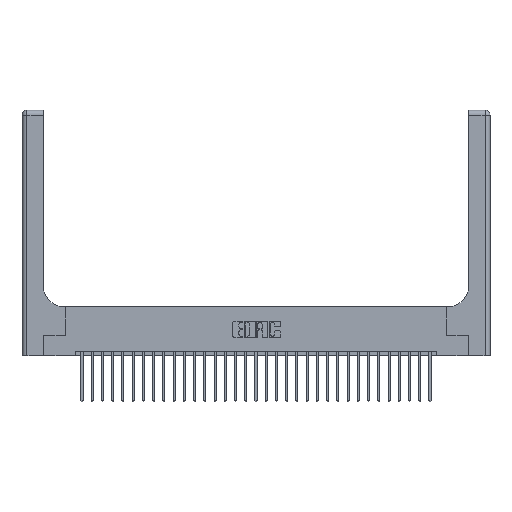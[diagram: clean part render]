
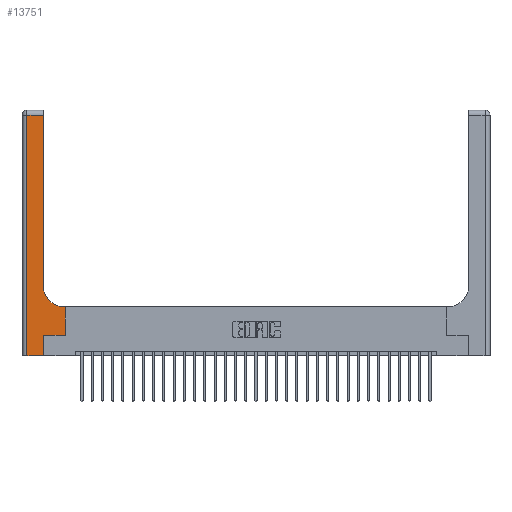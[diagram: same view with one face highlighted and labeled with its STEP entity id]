
A CAD part, top view. The second image highlights one B-rep face of the part: STEP entity #13751.
In plain terms, the highlighted planar face has unit normal (0, 0, 1).
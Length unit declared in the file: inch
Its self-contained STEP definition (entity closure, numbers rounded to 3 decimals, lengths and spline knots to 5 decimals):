
#212 = ORIENTED_EDGE ( 'NONE', *, *, #24034, .T. ) ;
#1287 = EDGE_CURVE ( 'NONE', #4562, #25562, #9006, .T. ) ;
#1289 = VERTEX_POINT ( 'NONE', #25247 ) ;
#1395 = LINE ( 'NONE', #23115, #12663 ) ;
#1479 = ORIENTED_EDGE ( 'NONE', *, *, #27696, .T. ) ;
#1590 = ORIENTED_EDGE ( 'NONE', *, *, #26799, .T. ) ;
#1836 = EDGE_CURVE ( 'NONE', #21965, #18299, #26508, .T. ) ;
#2202 = CARTESIAN_POINT ( 'NONE',  ( 0.265, 0.25, 0.37 ) ) ;
#2349 = CARTESIAN_POINT ( 'NONE',  ( 0.06, 3., 0.37 ) ) ;
#2582 = ORIENTED_EDGE ( 'NONE', *, *, #17520, .T. ) ;
#3623 = ORIENTED_EDGE ( 'NONE', *, *, #25007, .T. ) ;
#3646 = CARTESIAN_POINT ( 'NONE',  ( 0.26, 3., 0.37 ) ) ;
#4562 = VERTEX_POINT ( 'NONE', #13557 ) ;
#5045 = LINE ( 'NONE', #2202, #22227 ) ;
#6252 = VERTEX_POINT ( 'NONE', #26612 ) ;
#6631 = EDGE_CURVE ( 'NONE', #1289, #6252, #18852, .T. ) ;
#6701 = DIRECTION ( 'NONE',  ( -1., 0., 0. ) ) ;
#6970 = VERTEX_POINT ( 'NONE', #17589 ) ;
#7402 = VECTOR ( 'NONE', #24679, 39.37008 ) ;
#7722 = DIRECTION ( 'NONE',  ( -1., 0., 0. ) ) ;
#8381 = DIRECTION ( 'NONE',  ( 0., 1., 0. ) ) ;
#8874 = VECTOR ( 'NONE', #19565, 39.37008 ) ;
#9006 = LINE ( 'NONE', #11857, #16437 ) ;
#9438 = CARTESIAN_POINT ( 'NONE',  ( 0.06, 2.94, 0.37 ) ) ;
#9473 = CARTESIAN_POINT ( 'NONE',  ( 0.51, 0.6, 0.37 ) ) ;
#10012 = FACE_OUTER_BOUND ( 'NONE', #28015, .T. ) ;
#10617 = CARTESIAN_POINT ( 'NONE',  ( 0.528, 0.25, 0.37 ) ) ;
#10972 = CARTESIAN_POINT ( 'NONE',  ( 0., 2.94, 0.37 ) ) ;
#11434 = VECTOR ( 'NONE', #20041, 39.37008 ) ;
#11857 = CARTESIAN_POINT ( 'NONE',  ( 0.26, 0.6, 0.37 ) ) ;
#11878 = CIRCLE ( 'NONE', #12077, 0.25 ) ;
#11880 = CARTESIAN_POINT ( 'NONE',  ( 0.51, 0.85, 0.37 ) ) ;
#12077 = AXIS2_PLACEMENT_3D ( 'NONE', #11880, #16510, #27521 ) ;
#12663 = VECTOR ( 'NONE', #25536, 39.37008 ) ;
#13555 = LINE ( 'NONE', #3646, #11434 ) ;
#13557 = CARTESIAN_POINT ( 'NONE',  ( 0.528, 0.6, 0.37 ) ) ;
#13751 = ADVANCED_FACE ( 'NONE', ( #10012 ), #20365, .F. ) ;
#14446 = DIRECTION ( 'NONE',  ( -1., 0., 0. ) ) ;
#15959 = ORIENTED_EDGE ( 'NONE', *, *, #20061, .T. ) ;
#16300 = LINE ( 'NONE', #10617, #8874 ) ;
#16437 = VECTOR ( 'NONE', #7722, 39.37008 ) ;
#16510 = DIRECTION ( 'NONE',  ( 0., 0., -1. ) ) ;
#16699 = VERTEX_POINT ( 'NONE', #26173 ) ;
#17457 = VECTOR ( 'NONE', #14446, 39.37008 ) ;
#17520 = EDGE_CURVE ( 'NONE', #6252, #6970, #5045, .T. ) ;
#17589 = CARTESIAN_POINT ( 'NONE',  ( 0.528, 0.25, 0.37 ) ) ;
#17983 = ORIENTED_EDGE ( 'NONE', *, *, #1836, .T. ) ;
#18299 = VERTEX_POINT ( 'NONE', #9438 ) ;
#18852 = LINE ( 'NONE', #26395, #25436 ) ;
#19364 = LINE ( 'NONE', #2349, #7402 ) ;
#19565 = DIRECTION ( 'NONE',  ( 0., 1., 0. ) ) ;
#19853 = CARTESIAN_POINT ( 'NONE',  ( 0.26, 2.94, 0.37 ) ) ;
#20041 = DIRECTION ( 'NONE',  ( 0., 1., 0. ) ) ;
#20061 = EDGE_CURVE ( 'NONE', #18299, #20347, #19364, .T. ) ;
#20347 = VERTEX_POINT ( 'NONE', #22219 ) ;
#20365 = PLANE ( 'NONE',  #28896 ) ;
#20481 = DIRECTION ( 'NONE',  ( 1., 0., 0. ) ) ;
#21965 = VERTEX_POINT ( 'NONE', #19853 ) ;
#22219 = CARTESIAN_POINT ( 'NONE',  ( 0.06, 0., 0.37 ) ) ;
#22227 = VECTOR ( 'NONE', #20481, 39.37008 ) ;
#22677 = CARTESIAN_POINT ( 'NONE',  ( 0., 3., 0.37 ) ) ;
#23115 = CARTESIAN_POINT ( 'NONE',  ( 0., 0., 0.37 ) ) ;
#24034 = EDGE_CURVE ( 'NONE', #20347, #1289, #1395, .T. ) ;
#24679 = DIRECTION ( 'NONE',  ( 0., -1., 0. ) ) ;
#24915 = DIRECTION ( 'NONE',  ( 0., 0., -1. ) ) ;
#25007 = EDGE_CURVE ( 'NONE', #25562, #16699, #11878, .T. ) ;
#25247 = CARTESIAN_POINT ( 'NONE',  ( 0.265, 0., 0.37 ) ) ;
#25436 = VECTOR ( 'NONE', #8381, 39.37008 ) ;
#25536 = DIRECTION ( 'NONE',  ( 1., 0., 0. ) ) ;
#25562 = VERTEX_POINT ( 'NONE', #9473 ) ;
#25683 = ORIENTED_EDGE ( 'NONE', *, *, #6631, .T. ) ;
#26173 = CARTESIAN_POINT ( 'NONE',  ( 0.26, 0.85, 0.37 ) ) ;
#26395 = CARTESIAN_POINT ( 'NONE',  ( 0.265, 0., 0.37 ) ) ;
#26508 = LINE ( 'NONE', #10972, #17457 ) ;
#26612 = CARTESIAN_POINT ( 'NONE',  ( 0.265, 0.25, 0.37 ) ) ;
#26799 = EDGE_CURVE ( 'NONE', #16699, #21965, #13555, .T. ) ;
#27521 = DIRECTION ( 'NONE',  ( 1., 0., 0. ) ) ;
#27696 = EDGE_CURVE ( 'NONE', #6970, #4562, #16300, .T. ) ;
#27782 = ORIENTED_EDGE ( 'NONE', *, *, #1287, .T. ) ;
#28015 = EDGE_LOOP ( 'NONE', ( #1590, #17983, #15959, #212, #25683, #2582, #1479, #27782, #3623 ) ) ;
#28896 = AXIS2_PLACEMENT_3D ( 'NONE', #22677, #24915, #6701 ) ;
